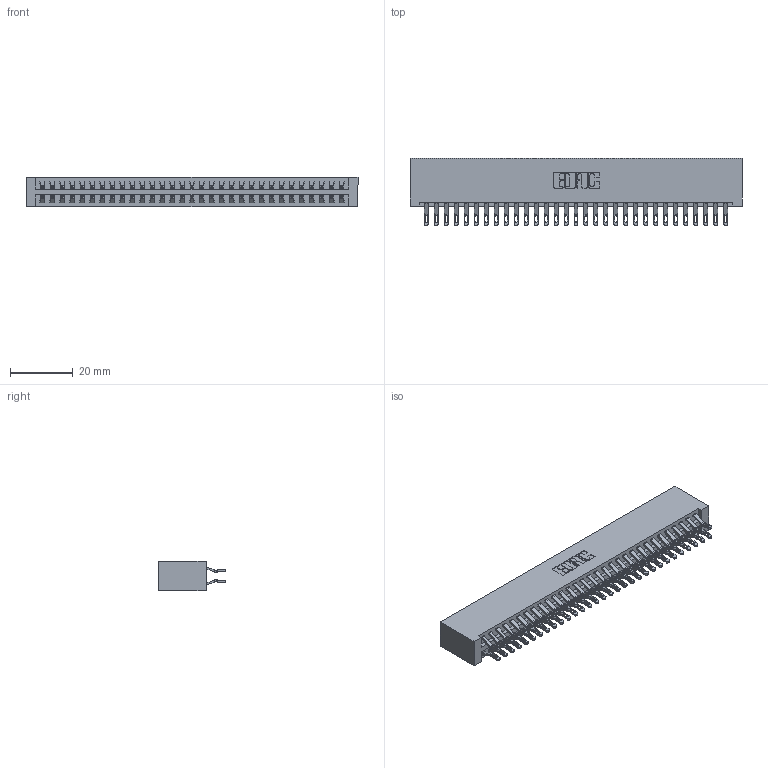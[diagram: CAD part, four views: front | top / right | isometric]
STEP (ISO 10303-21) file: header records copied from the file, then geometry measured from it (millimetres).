
FILE_DESCRIPTION (( 'STEP AP203' ), '1' );
FILE_NAME ('396-062-555-201.STEP', '2018-09-08T15:27:34', ( '' ), ( '' ), 'SwSTEP 2.0', 'SolidWorks 2016', '' );
FILE_SCHEMA (( 'CONFIG_CONTROL_DESIGN' ));
Length unit declared in the file: inch
Products named in the file (3): 345-292-001_555 Tail; 396-062-555-201; 346 Part_No Mounting Lugs
Assembly tree (63 placements, depth 2):
  396-062-555-201
    346 Part_No Mounting Lugs
    345-292-001_555 Tail  x62
Bounding box: 105.66 x 21.46 x 9.4 mm (x, y, z)
Volume: 10971.2 mm3; surface area: 15712 mm2
Topology: 63 solids, 63 shells, 3710 faces, 11651 edges, 7766 vertices
Faces by surface type: plane 2118, cylinder 1592
Entity records: 21761 total; most frequent: CARTESIAN_POINT 3634, ORIENTED_EDGE 3538, DIRECTION 3217, EDGE_CURVE 1769, LINE 1501, VECTOR 1501, VERTEX_POINT 1178, AXIS2_PLACEMENT_3D 858
